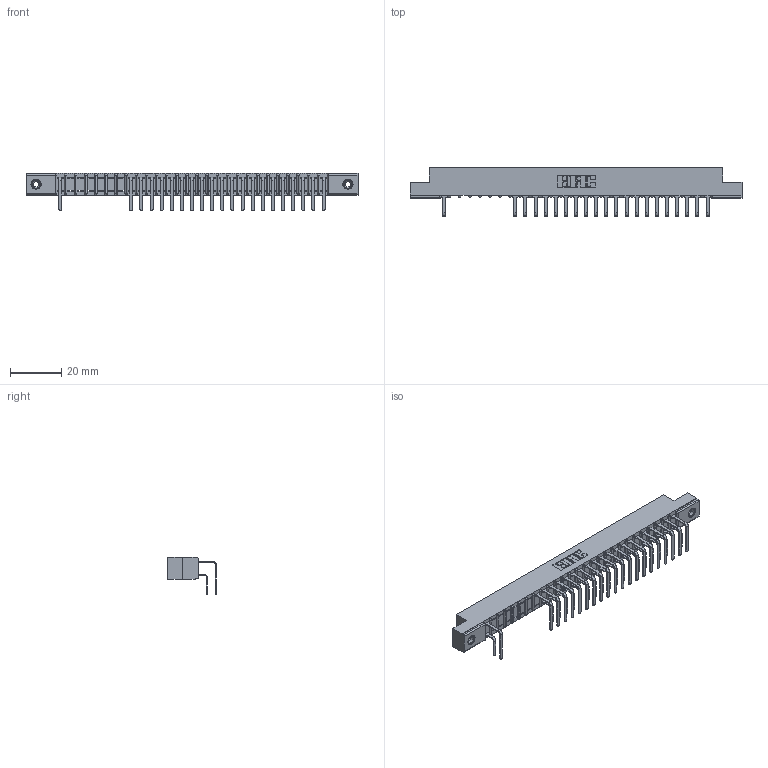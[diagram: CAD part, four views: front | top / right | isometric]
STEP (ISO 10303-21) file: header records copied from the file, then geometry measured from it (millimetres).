
FILE_DESCRIPTION (( 'STEP AP203' ), '1' );
FILE_NAME ('357-027-558-108.STEP', '2018-08-09T04:37:45', ( '' ), ( '' ), 'SwSTEP 2.0', 'SolidWorks 2016', '' );
FILE_SCHEMA (( 'CONFIG_CONTROL_DESIGN' ));
Length unit declared in the file: inch
Products named in the file (5): 345-250-001_345-250-003-102; 357-027-558-108; 307 Part_.156 Dia Mounting Holes; 307-290-001_558 559 - 1 (Single); 307-290-001_558 - 2 (Single)
Assembly tree (44 placements, depth 2):
  357-027-558-108
    307 Part_.156 Dia Mounting Holes
    307-290-001_558 559 - 1 (Single)  x20
    307-290-001_558 - 2 (Single)  x21
    345-250-001_345-250-003-102  x2
Bounding box: 130 x 18.96 x 14.81 mm (x, y, z)
Volume: 8511.2 mm3; surface area: 15354.5 mm2
Topology: 44 solids, 44 shells, 2386 faces, 6697 edges, 4326 vertices
Faces by surface type: plane 1533, cylinder 781, sphere 56, cone 12, torus 4
Entity records: 28076 total; most frequent: CARTESIAN_POINT 4639, ORIENTED_EDGE 4602, DIRECTION 4545, EDGE_CURVE 2301, VECTOR 1757, LINE 1757, VERTEX_POINT 1488, AXIS2_PLACEMENT_3D 1394
